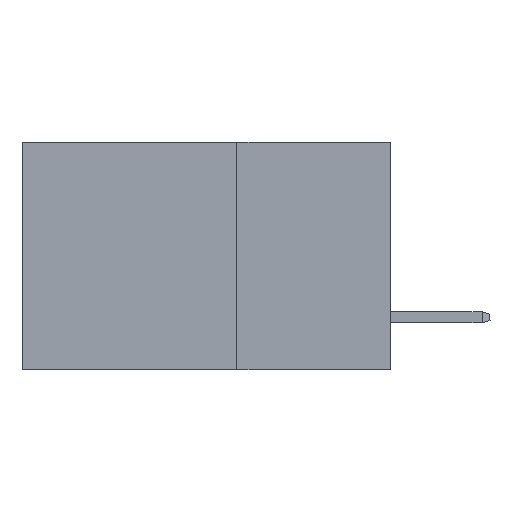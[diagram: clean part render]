
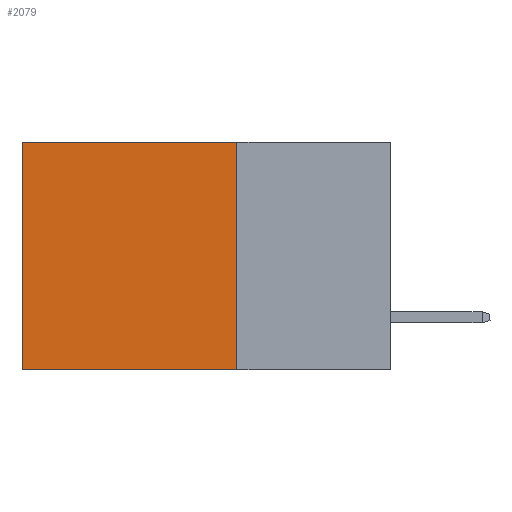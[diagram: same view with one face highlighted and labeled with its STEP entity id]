
A CAD part, left-side view. The second image highlights one B-rep face of the part: STEP entity #2079.
In plain terms, the highlighted planar face has unit normal (-1, 0, 0).
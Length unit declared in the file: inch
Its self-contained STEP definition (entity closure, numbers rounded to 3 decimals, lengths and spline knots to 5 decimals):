
#914 = EDGE_LOOP ( 'NONE', ( #30420, #24434, #26451, #20667 ) ) ;
#2079 = ADVANCED_FACE ( 'NONE', ( #4268 ), #23487, .F. ) ;
#2463 = LINE ( 'NONE', #18831, #16677 ) ;
#4268 = FACE_OUTER_BOUND ( 'NONE', #914, .T. ) ;
#4529 = CARTESIAN_POINT ( 'NONE',  ( 0.2875, 0.6, 0. ) ) ;
#5318 = CARTESIAN_POINT ( 'NONE',  ( 0.2875, 0.25, 0. ) ) ;
#5829 = LINE ( 'NONE', #31450, #20748 ) ;
#9486 = DIRECTION ( 'NONE',  ( 0., 0., -1. ) ) ;
#10726 = EDGE_CURVE ( 'NONE', #28834, #13535, #21834, .T. ) ;
#11514 = CARTESIAN_POINT ( 'NONE',  ( 0.2875, 0.6, -0.37 ) ) ;
#13344 = DIRECTION ( 'NONE',  ( 0., 1., 0. ) ) ;
#13535 = VERTEX_POINT ( 'NONE', #4529 ) ;
#15390 = LINE ( 'NONE', #18786, #29083 ) ;
#16677 = VECTOR ( 'NONE', #13344, 39.37008 ) ;
#18373 = VERTEX_POINT ( 'NONE', #11514 ) ;
#18786 = CARTESIAN_POINT ( 'NONE',  ( 0.2875, 0.25, 0. ) ) ;
#18831 = CARTESIAN_POINT ( 'NONE',  ( 0.2875, 0.25, -0.37 ) ) ;
#18908 = DIRECTION ( 'NONE',  ( 0., 0., -1. ) ) ;
#19351 = CARTESIAN_POINT ( 'NONE',  ( 0.2875, 0.25, 0. ) ) ;
#19430 = CARTESIAN_POINT ( 'NONE',  ( 0.2875, 0.25, -0.37 ) ) ;
#20667 = ORIENTED_EDGE ( 'NONE', *, *, #10726, .T. ) ;
#20748 = VECTOR ( 'NONE', #9486, 39.37008 ) ;
#21834 = LINE ( 'NONE', #5318, #28199 ) ;
#22401 = AXIS2_PLACEMENT_3D ( 'NONE', #23634, #23747, #33752 ) ;
#22415 = VERTEX_POINT ( 'NONE', #19430 ) ;
#23487 = PLANE ( 'NONE',  #22401 ) ;
#23634 = CARTESIAN_POINT ( 'NONE',  ( 0.2875, 0.25, 0. ) ) ;
#23747 = DIRECTION ( 'NONE',  ( 1., 0., 0. ) ) ;
#24434 = ORIENTED_EDGE ( 'NONE', *, *, #31245, .F. ) ;
#25140 = EDGE_CURVE ( 'NONE', #28834, #22415, #15390, .T. ) ;
#26451 = ORIENTED_EDGE ( 'NONE', *, *, #25140, .F. ) ;
#27560 = DIRECTION ( 'NONE',  ( 0., 1., 0. ) ) ;
#28199 = VECTOR ( 'NONE', #27560, 39.37008 ) ;
#28834 = VERTEX_POINT ( 'NONE', #19351 ) ;
#29083 = VECTOR ( 'NONE', #18908, 39.37008 ) ;
#30420 = ORIENTED_EDGE ( 'NONE', *, *, #35202, .T. ) ;
#31245 = EDGE_CURVE ( 'NONE', #22415, #18373, #2463, .T. ) ;
#31450 = CARTESIAN_POINT ( 'NONE',  ( 0.2875, 0.6, 0. ) ) ;
#33752 = DIRECTION ( 'NONE',  ( 0., 0., -1. ) ) ;
#35202 = EDGE_CURVE ( 'NONE', #13535, #18373, #5829, .T. ) ;
